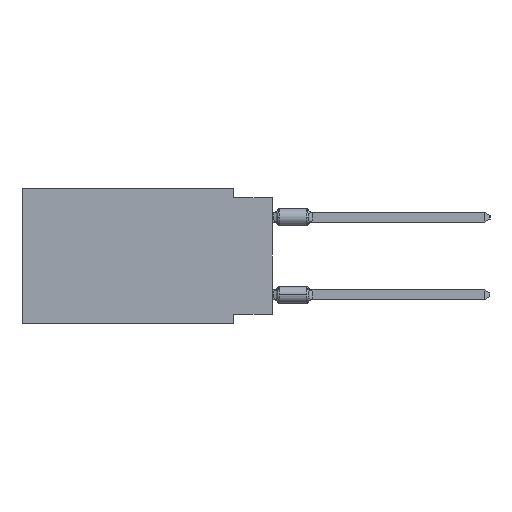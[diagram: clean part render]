
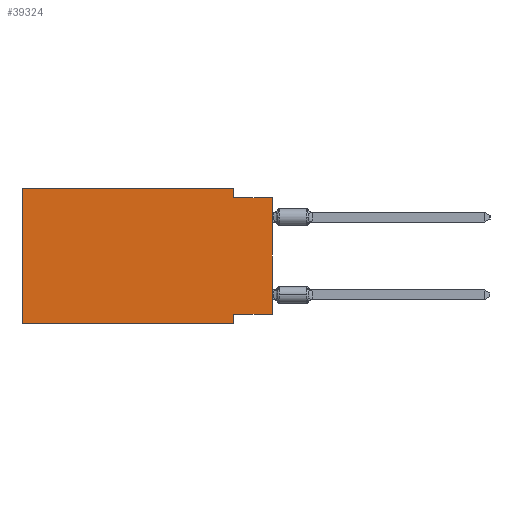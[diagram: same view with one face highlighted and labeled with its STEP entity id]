
A CAD part, left-side view. The second image highlights one B-rep face of the part: STEP entity #39324.
In plain terms, the highlighted planar face has unit normal (-1, 0, 0).
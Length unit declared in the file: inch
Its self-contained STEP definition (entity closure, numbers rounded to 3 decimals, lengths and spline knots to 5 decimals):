
#366 = VERTEX_POINT ( 'NONE', #41830 ) ;
#1171 = CARTESIAN_POINT ( 'NONE',  ( 0., 0., -0.025 ) ) ;
#1212 = ORIENTED_EDGE ( 'NONE', *, *, #11343, .F. ) ;
#2477 = ORIENTED_EDGE ( 'NONE', *, *, #14548, .F. ) ;
#3314 = CARTESIAN_POINT ( 'NONE',  ( 0., 0., -0.325 ) ) ;
#3587 = EDGE_CURVE ( 'NONE', #30563, #34223, #15785, .T. ) ;
#3604 = VERTEX_POINT ( 'NONE', #5665 ) ;
#3775 = VECTOR ( 'NONE', #15560, 39.37008 ) ;
#4376 = CARTESIAN_POINT ( 'NONE',  ( 0., 0.1, -0.025 ) ) ;
#5665 = CARTESIAN_POINT ( 'NONE',  ( 0., 0.645, -0.35 ) ) ;
#7117 = CARTESIAN_POINT ( 'NONE',  ( 0., 0.645, 0. ) ) ;
#7228 = VERTEX_POINT ( 'NONE', #43795 ) ;
#8123 = ORIENTED_EDGE ( 'NONE', *, *, #41503, .F. ) ;
#8384 = LINE ( 'NONE', #18712, #35217 ) ;
#11245 = FACE_OUTER_BOUND ( 'NONE', #32911, .T. ) ;
#11343 = EDGE_CURVE ( 'NONE', #7228, #366, #8384, .T. ) ;
#11612 = ORIENTED_EDGE ( 'NONE', *, *, #37197, .T. ) ;
#11904 = VERTEX_POINT ( 'NONE', #29642 ) ;
#12475 = LINE ( 'NONE', #40406, #24462 ) ;
#12538 = EDGE_CURVE ( 'NONE', #11904, #7228, #44965, .T. ) ;
#13657 = CARTESIAN_POINT ( 'NONE',  ( 0., 0.645, 0. ) ) ;
#14095 = LINE ( 'NONE', #24850, #21284 ) ;
#14488 = EDGE_CURVE ( 'NONE', #3604, #19923, #12475, .T. ) ;
#14513 = DIRECTION ( 'NONE',  ( 0., 1., 0. ) ) ;
#14548 = EDGE_CURVE ( 'NONE', #34223, #44625, #21311, .T. ) ;
#15272 = DIRECTION ( 'NONE',  ( 0., 0., -1. ) ) ;
#15560 = DIRECTION ( 'NONE',  ( 0., 0., -1. ) ) ;
#15785 = LINE ( 'NONE', #43468, #3775 ) ;
#16381 = DIRECTION ( 'NONE',  ( 0., -1., 0. ) ) ;
#17218 = CARTESIAN_POINT ( 'NONE',  ( 0., 0., 0. ) ) ;
#17674 = DIRECTION ( 'NONE',  ( 1., 0., 0. ) ) ;
#18712 = CARTESIAN_POINT ( 'NONE',  ( 0., 0.1, -0.35 ) ) ;
#19403 = ORIENTED_EDGE ( 'NONE', *, *, #14488, .F. ) ;
#19732 = ORIENTED_EDGE ( 'NONE', *, *, #3587, .F. ) ;
#19923 = VERTEX_POINT ( 'NONE', #13657 ) ;
#19990 = VECTOR ( 'NONE', #14513, 39.37008 ) ;
#20864 = DIRECTION ( 'NONE',  ( 0., 0., 1. ) ) ;
#21284 = VECTOR ( 'NONE', #28062, 39.37008 ) ;
#21311 = LINE ( 'NONE', #1171, #42047 ) ;
#21990 = PLANE ( 'NONE',  #34261 ) ;
#23144 = CARTESIAN_POINT ( 'NONE',  ( 0., 0., -0.025 ) ) ;
#23774 = VECTOR ( 'NONE', #20864, 39.37008 ) ;
#24462 = VECTOR ( 'NONE', #37428, 39.37008 ) ;
#24850 = CARTESIAN_POINT ( 'NONE',  ( 0., 0.645, 0. ) ) ;
#26671 = LINE ( 'NONE', #33768, #39548 ) ;
#28062 = DIRECTION ( 'NONE',  ( 0., -1., 0. ) ) ;
#29231 = EDGE_CURVE ( 'NONE', #11904, #44625, #30706, .T. ) ;
#29642 = CARTESIAN_POINT ( 'NONE',  ( 0., 0., -0.325 ) ) ;
#30563 = VERTEX_POINT ( 'NONE', #42284 ) ;
#30706 = LINE ( 'NONE', #17218, #23774 ) ;
#31138 = ORIENTED_EDGE ( 'NONE', *, *, #29231, .T. ) ;
#32272 = DIRECTION ( 'NONE',  ( 0., -1., 0. ) ) ;
#32911 = EDGE_LOOP ( 'NONE', ( #31138, #2477, #19732, #8123, #19403, #11612, #1212, #41854 ) ) ;
#33768 = CARTESIAN_POINT ( 'NONE',  ( 0., 0.645, -0.35 ) ) ;
#34223 = VERTEX_POINT ( 'NONE', #4376 ) ;
#34261 = AXIS2_PLACEMENT_3D ( 'NONE', #7117, #17674, #35966 ) ;
#35217 = VECTOR ( 'NONE', #15272, 39.37008 ) ;
#35966 = DIRECTION ( 'NONE',  ( 0., 0., -1. ) ) ;
#37197 = EDGE_CURVE ( 'NONE', #3604, #366, #26671, .T. ) ;
#37428 = DIRECTION ( 'NONE',  ( 0., 0., 1. ) ) ;
#39324 = ADVANCED_FACE ( 'NONE', ( #11245 ), #21990, .F. ) ;
#39548 = VECTOR ( 'NONE', #16381, 39.37008 ) ;
#40406 = CARTESIAN_POINT ( 'NONE',  ( 0., 0.645, 0. ) ) ;
#41503 = EDGE_CURVE ( 'NONE', #19923, #30563, #14095, .T. ) ;
#41830 = CARTESIAN_POINT ( 'NONE',  ( 0., 0.1, -0.35 ) ) ;
#41854 = ORIENTED_EDGE ( 'NONE', *, *, #12538, .F. ) ;
#42047 = VECTOR ( 'NONE', #32272, 39.37008 ) ;
#42284 = CARTESIAN_POINT ( 'NONE',  ( 0., 0.1, 0. ) ) ;
#43468 = CARTESIAN_POINT ( 'NONE',  ( 0., 0.1, 0. ) ) ;
#43795 = CARTESIAN_POINT ( 'NONE',  ( 0., 0.1, -0.325 ) ) ;
#44625 = VERTEX_POINT ( 'NONE', #23144 ) ;
#44965 = LINE ( 'NONE', #3314, #19990 ) ;
